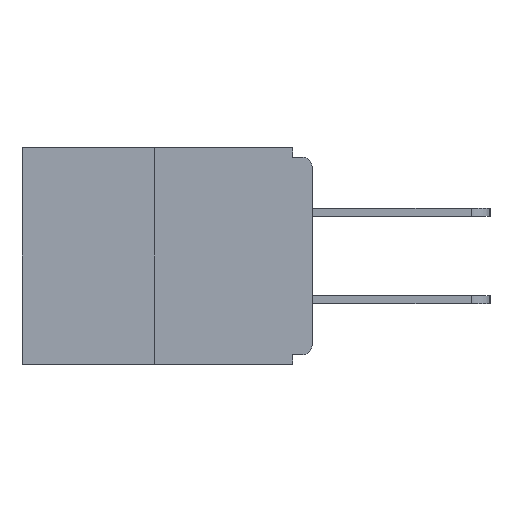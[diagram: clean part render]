
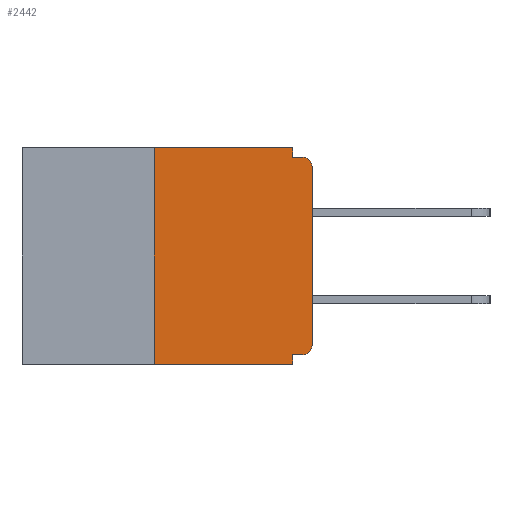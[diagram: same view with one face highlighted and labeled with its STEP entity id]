
A CAD part, left-side view. The second image highlights one B-rep face of the part: STEP entity #2442.
In plain terms, the highlighted planar face has unit normal (-1, 0, 0).
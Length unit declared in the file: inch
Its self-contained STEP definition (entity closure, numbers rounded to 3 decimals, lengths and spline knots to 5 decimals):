
#107 = ORIENTED_EDGE ( 'NONE', *, *, #4375, .T. ) ;
#177 = DIRECTION ( 'NONE',  ( -1., 0., 0. ) ) ;
#646 = DIRECTION ( 'NONE',  ( 0., -1., 0. ) ) ;
#823 = EDGE_CURVE ( 'NONE', #19174, #9057, #18385, .T. ) ;
#2155 = ORIENTED_EDGE ( 'NONE', *, *, #4879, .F. ) ;
#2164 = CARTESIAN_POINT ( 'NONE',  ( 0., 0.031, 0. ) ) ;
#2365 = CARTESIAN_POINT ( 'NONE',  ( 0., 0.015, -0.328 ) ) ;
#2439 = ORIENTED_EDGE ( 'NONE', *, *, #3357, .T. ) ;
#2442 = ADVANCED_FACE ( 'NONE', ( #19677 ), #16944, .F. ) ;
#2487 = CARTESIAN_POINT ( 'NONE',  ( 0., 0., -0.328 ) ) ;
#3040 = CARTESIAN_POINT ( 'NONE',  ( 0., 0.031, -0.343 ) ) ;
#3357 = EDGE_CURVE ( 'NONE', #14311, #3670, #21895, .T. ) ;
#3436 = CARTESIAN_POINT ( 'NONE',  ( 0., 0.031, 0. ) ) ;
#3670 = VERTEX_POINT ( 'NONE', #4697 ) ;
#4242 = EDGE_CURVE ( 'NONE', #12156, #6676, #20206, .T. ) ;
#4322 = VECTOR ( 'NONE', #14032, 39.37008 ) ;
#4375 = EDGE_CURVE ( 'NONE', #23110, #9057, #21552, .T. ) ;
#4697 = CARTESIAN_POINT ( 'NONE',  ( 0., 0., -0.03 ) ) ;
#4879 = EDGE_CURVE ( 'NONE', #9673, #19174, #17552, .T. ) ;
#5022 = AXIS2_PLACEMENT_3D ( 'NONE', #12439, #27029, #16759 ) ;
#5605 = DIRECTION ( 'NONE',  ( 0., 0., 1. ) ) ;
#5786 = CIRCLE ( 'NONE', #5022, 0.015 ) ;
#5931 = VECTOR ( 'NONE', #646, 39.37008 ) ;
#6427 = EDGE_CURVE ( 'NONE', #9673, #14311, #22412, .T. ) ;
#6676 = VERTEX_POINT ( 'NONE', #22571 ) ;
#7674 = DIRECTION ( 'NONE',  ( 0., 0., -1. ) ) ;
#7733 = LINE ( 'NONE', #3436, #8091 ) ;
#7774 = CARTESIAN_POINT ( 'NONE',  ( 0., 0.25, -0.343 ) ) ;
#8091 = VECTOR ( 'NONE', #7674, 39.37008 ) ;
#9057 = VERTEX_POINT ( 'NONE', #10574 ) ;
#9673 = VERTEX_POINT ( 'NONE', #2365 ) ;
#10207 = CARTESIAN_POINT ( 'NONE',  ( 0., 0.46, 0. ) ) ;
#10529 = VECTOR ( 'NONE', #5605, 39.37008 ) ;
#10574 = CARTESIAN_POINT ( 'NONE',  ( 0., 0.031, -0.343 ) ) ;
#12156 = VERTEX_POINT ( 'NONE', #18933 ) ;
#12439 = CARTESIAN_POINT ( 'NONE',  ( 0., 0.015, -0.03 ) ) ;
#13136 = CARTESIAN_POINT ( 'NONE',  ( 0., 0.015, -0.313 ) ) ;
#13720 = VERTEX_POINT ( 'NONE', #16299 ) ;
#14032 = DIRECTION ( 'NONE',  ( 0., 0., 1. ) ) ;
#14053 = EDGE_CURVE ( 'NONE', #16313, #12156, #7733, .T. ) ;
#14311 = VERTEX_POINT ( 'NONE', #23612 ) ;
#14387 = AXIS2_PLACEMENT_3D ( 'NONE', #13136, #177, #17155 ) ;
#14526 = LINE ( 'NONE', #16195, #10529 ) ;
#15467 = LINE ( 'NONE', #21640, #21762 ) ;
#15632 = EDGE_CURVE ( 'NONE', #23110, #13720, #14526, .T. ) ;
#16195 = CARTESIAN_POINT ( 'NONE',  ( 0., 0.25, 0. ) ) ;
#16299 = CARTESIAN_POINT ( 'NONE',  ( 0., 0.25, 0. ) ) ;
#16313 = VERTEX_POINT ( 'NONE', #2164 ) ;
#16759 = DIRECTION ( 'NONE',  ( 0., 0., -1. ) ) ;
#16915 = VECTOR ( 'NONE', #23670, 39.37008 ) ;
#16944 = PLANE ( 'NONE',  #24100 ) ;
#17155 = DIRECTION ( 'NONE',  ( 0., 0., -1. ) ) ;
#17552 = LINE ( 'NONE', #2487, #17847 ) ;
#17642 = EDGE_CURVE ( 'NONE', #3670, #6676, #5786, .T. ) ;
#17664 = ORIENTED_EDGE ( 'NONE', *, *, #17642, .T. ) ;
#17847 = VECTOR ( 'NONE', #19095, 39.37008 ) ;
#18385 = LINE ( 'NONE', #3040, #21729 ) ;
#18933 = CARTESIAN_POINT ( 'NONE',  ( 0., 0.031, -0.015 ) ) ;
#19095 = DIRECTION ( 'NONE',  ( 0., 1., 0. ) ) ;
#19174 = VERTEX_POINT ( 'NONE', #27020 ) ;
#19208 = ORIENTED_EDGE ( 'NONE', *, *, #4242, .F. ) ;
#19677 = FACE_OUTER_BOUND ( 'NONE', #25224, .T. ) ;
#20206 = LINE ( 'NONE', #23754, #5931 ) ;
#20608 = ORIENTED_EDGE ( 'NONE', *, *, #23590, .F. ) ;
#21107 = DIRECTION ( 'NONE',  ( 0., 0., -1. ) ) ;
#21552 = LINE ( 'NONE', #21804, #16915 ) ;
#21640 = CARTESIAN_POINT ( 'NONE',  ( 0., 0.46, 0. ) ) ;
#21729 = VECTOR ( 'NONE', #21965, 39.37008 ) ;
#21762 = VECTOR ( 'NONE', #23409, 39.37008 ) ;
#21804 = CARTESIAN_POINT ( 'NONE',  ( 0., 0.46, -0.343 ) ) ;
#21895 = LINE ( 'NONE', #24523, #4322 ) ;
#21965 = DIRECTION ( 'NONE',  ( 0., 0., -1. ) ) ;
#22412 = CIRCLE ( 'NONE', #14387, 0.015 ) ;
#22571 = CARTESIAN_POINT ( 'NONE',  ( 0., 0.015, -0.015 ) ) ;
#23046 = ORIENTED_EDGE ( 'NONE', *, *, #6427, .T. ) ;
#23110 = VERTEX_POINT ( 'NONE', #7774 ) ;
#23409 = DIRECTION ( 'NONE',  ( 0., -1., 0. ) ) ;
#23485 = ORIENTED_EDGE ( 'NONE', *, *, #15632, .F. ) ;
#23590 = EDGE_CURVE ( 'NONE', #13720, #16313, #15467, .T. ) ;
#23612 = CARTESIAN_POINT ( 'NONE',  ( 0., 0., -0.313 ) ) ;
#23661 = ORIENTED_EDGE ( 'NONE', *, *, #823, .F. ) ;
#23670 = DIRECTION ( 'NONE',  ( 0., -1., 0. ) ) ;
#23754 = CARTESIAN_POINT ( 'NONE',  ( 0., 0., -0.015 ) ) ;
#24100 = AXIS2_PLACEMENT_3D ( 'NONE', #10207, #27221, #21107 ) ;
#24523 = CARTESIAN_POINT ( 'NONE',  ( 0., 0., 0. ) ) ;
#25224 = EDGE_LOOP ( 'NONE', ( #20608, #23485, #107, #23661, #2155, #23046, #2439, #17664, #19208, #27327 ) ) ;
#27020 = CARTESIAN_POINT ( 'NONE',  ( 0., 0.031, -0.328 ) ) ;
#27029 = DIRECTION ( 'NONE',  ( -1., 0., 0. ) ) ;
#27221 = DIRECTION ( 'NONE',  ( 1., 0., 0. ) ) ;
#27327 = ORIENTED_EDGE ( 'NONE', *, *, #14053, .F. ) ;
